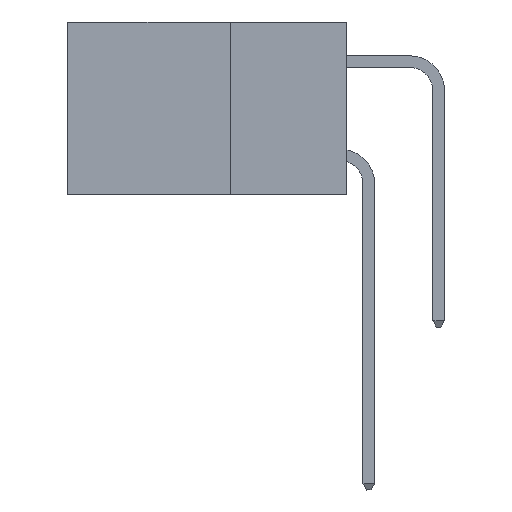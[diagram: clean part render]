
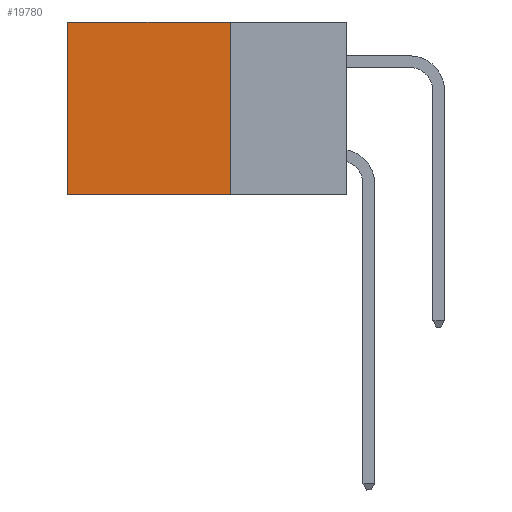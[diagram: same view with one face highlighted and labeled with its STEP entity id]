
A CAD part, left-side view. The second image highlights one B-rep face of the part: STEP entity #19780.
In plain terms, the highlighted planar face has unit normal (-1, 0, 0).
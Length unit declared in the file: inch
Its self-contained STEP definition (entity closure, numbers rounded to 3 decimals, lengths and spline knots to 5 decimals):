
#30 = ORIENTED_EDGE ( 'NONE', *, *, #20375, .F. ) ;
#264 = EDGE_CURVE ( 'NONE', #6409, #15628, #20940, .T. ) ;
#335 = VERTEX_POINT ( 'NONE', #10973 ) ;
#813 = DIRECTION ( 'NONE',  ( 0., 1., 0. ) ) ;
#1534 = CARTESIAN_POINT ( 'NONE',  ( 0.2875, 0.25, 0. ) ) ;
#2327 = VERTEX_POINT ( 'NONE', #26992 ) ;
#3565 = EDGE_CURVE ( 'NONE', #2327, #15628, #12080, .T. ) ;
#3570 = PLANE ( 'NONE',  #18180 ) ;
#3776 = FACE_OUTER_BOUND ( 'NONE', #12432, .T. ) ;
#4147 = CARTESIAN_POINT ( 'NONE',  ( 0.2875, 0.6, 0. ) ) ;
#5101 = ORIENTED_EDGE ( 'NONE', *, *, #3565, .F. ) ;
#5190 = VECTOR ( 'NONE', #813, 39.37008 ) ;
#6409 = VERTEX_POINT ( 'NONE', #4147 ) ;
#7961 = VECTOR ( 'NONE', #17218, 39.37008 ) ;
#8291 = LINE ( 'NONE', #14449, #7961 ) ;
#10332 = DIRECTION ( 'NONE',  ( 0., 1., 0. ) ) ;
#10973 = CARTESIAN_POINT ( 'NONE',  ( 0.2875, 0.25, 0. ) ) ;
#12080 = LINE ( 'NONE', #23702, #16949 ) ;
#12163 = ORIENTED_EDGE ( 'NONE', *, *, #264, .T. ) ;
#12432 = EDGE_LOOP ( 'NONE', ( #12163, #5101, #30, #26996 ) ) ;
#13498 = EDGE_CURVE ( 'NONE', #335, #6409, #23011, .T. ) ;
#14449 = CARTESIAN_POINT ( 'NONE',  ( 0.2875, 0.25, 0. ) ) ;
#15628 = VERTEX_POINT ( 'NONE', #27516 ) ;
#16784 = DIRECTION ( 'NONE',  ( 1., 0., 0. ) ) ;
#16949 = VECTOR ( 'NONE', #10332, 39.37008 ) ;
#17218 = DIRECTION ( 'NONE',  ( 0., 0., -1. ) ) ;
#18180 = AXIS2_PLACEMENT_3D ( 'NONE', #1534, #16784, #19223 ) ;
#19223 = DIRECTION ( 'NONE',  ( 0., 0., -1. ) ) ;
#19466 = DIRECTION ( 'NONE',  ( 0., 0., -1. ) ) ;
#19780 = ADVANCED_FACE ( 'NONE', ( #3776 ), #3570, .F. ) ;
#20375 = EDGE_CURVE ( 'NONE', #335, #2327, #8291, .T. ) ;
#20940 = LINE ( 'NONE', #25899, #23741 ) ;
#23011 = LINE ( 'NONE', #27506, #5190 ) ;
#23702 = CARTESIAN_POINT ( 'NONE',  ( 0.2875, 0.25, -0.37 ) ) ;
#23741 = VECTOR ( 'NONE', #19466, 39.37008 ) ;
#25899 = CARTESIAN_POINT ( 'NONE',  ( 0.2875, 0.6, 0. ) ) ;
#26992 = CARTESIAN_POINT ( 'NONE',  ( 0.2875, 0.25, -0.37 ) ) ;
#26996 = ORIENTED_EDGE ( 'NONE', *, *, #13498, .T. ) ;
#27506 = CARTESIAN_POINT ( 'NONE',  ( 0.2875, 0.25, 0. ) ) ;
#27516 = CARTESIAN_POINT ( 'NONE',  ( 0.2875, 0.6, -0.37 ) ) ;
